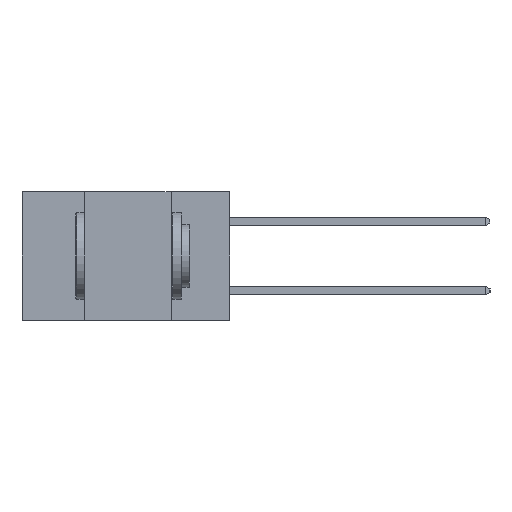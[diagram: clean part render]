
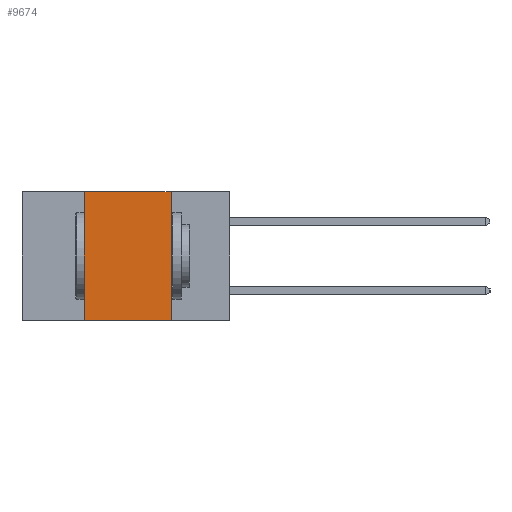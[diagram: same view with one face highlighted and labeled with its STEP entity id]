
A CAD part, left-side view. The second image highlights one B-rep face of the part: STEP entity #9674.
In plain terms, the highlighted planar face has unit normal (-1, 0, 0).
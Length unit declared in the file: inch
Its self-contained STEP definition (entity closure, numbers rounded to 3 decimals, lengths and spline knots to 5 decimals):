
#28 = EDGE_CURVE ( 'NONE', #226, #3965, #865, .T. ) ;
#223 = DIRECTION ( 'NONE',  ( 0., -1., 0. ) ) ;
#226 = VERTEX_POINT ( 'NONE', #11473 ) ;
#334 = EDGE_CURVE ( 'NONE', #10805, #3965, #4569, .T. ) ;
#865 = LINE ( 'NONE', #4439, #7903 ) ;
#2763 = CARTESIAN_POINT ( 'NONE',  ( 0., 0.42, 0. ) ) ;
#3119 = VECTOR ( 'NONE', #223, 39.37008 ) ;
#3965 = VERTEX_POINT ( 'NONE', #6001 ) ;
#4199 = CARTESIAN_POINT ( 'NONE',  ( 0., 0.42, -0.37 ) ) ;
#4238 = PLANE ( 'NONE',  #6480 ) ;
#4261 = VECTOR ( 'NONE', #9005, 39.37008 ) ;
#4439 = CARTESIAN_POINT ( 'NONE',  ( 0., 0.6, -0.37 ) ) ;
#4569 = LINE ( 'NONE', #5300, #4261 ) ;
#4971 = EDGE_LOOP ( 'NONE', ( #5362, #8243, #6573, #6876 ) ) ;
#5300 = CARTESIAN_POINT ( 'NONE',  ( 0., 0.17, -0.37 ) ) ;
#5362 = ORIENTED_EDGE ( 'NONE', *, *, #334, .F. ) ;
#5651 = LINE ( 'NONE', #10680, #3119 ) ;
#6001 = CARTESIAN_POINT ( 'NONE',  ( 0., 0.17, -0.37 ) ) ;
#6181 = DIRECTION ( 'NONE',  ( 0., 0., -1. ) ) ;
#6412 = FACE_OUTER_BOUND ( 'NONE', #4971, .T. ) ;
#6480 = AXIS2_PLACEMENT_3D ( 'NONE', #10967, #11947, #6181 ) ;
#6573 = ORIENTED_EDGE ( 'NONE', *, *, #11310, .F. ) ;
#6876 = ORIENTED_EDGE ( 'NONE', *, *, #28, .T. ) ;
#7290 = LINE ( 'NONE', #4199, #11193 ) ;
#7903 = VECTOR ( 'NONE', #9115, 39.37008 ) ;
#8243 = ORIENTED_EDGE ( 'NONE', *, *, #9533, .F. ) ;
#9005 = DIRECTION ( 'NONE',  ( 0., 0., -1. ) ) ;
#9023 = CARTESIAN_POINT ( 'NONE',  ( 0., 0.17, 0. ) ) ;
#9115 = DIRECTION ( 'NONE',  ( 0., -1., 0. ) ) ;
#9314 = VERTEX_POINT ( 'NONE', #2763 ) ;
#9533 = EDGE_CURVE ( 'NONE', #9314, #10805, #5651, .T. ) ;
#9674 = ADVANCED_FACE ( 'NONE', ( #6412 ), #4238, .F. ) ;
#10680 = CARTESIAN_POINT ( 'NONE',  ( 0., 0.6, 0. ) ) ;
#10805 = VERTEX_POINT ( 'NONE', #9023 ) ;
#10893 = DIRECTION ( 'NONE',  ( 0., 0., 1. ) ) ;
#10967 = CARTESIAN_POINT ( 'NONE',  ( 0., 0.6, 0. ) ) ;
#11193 = VECTOR ( 'NONE', #10893, 39.37008 ) ;
#11310 = EDGE_CURVE ( 'NONE', #226, #9314, #7290, .T. ) ;
#11473 = CARTESIAN_POINT ( 'NONE',  ( 0., 0.42, -0.37 ) ) ;
#11947 = DIRECTION ( 'NONE',  ( 1., 0., 0. ) ) ;
